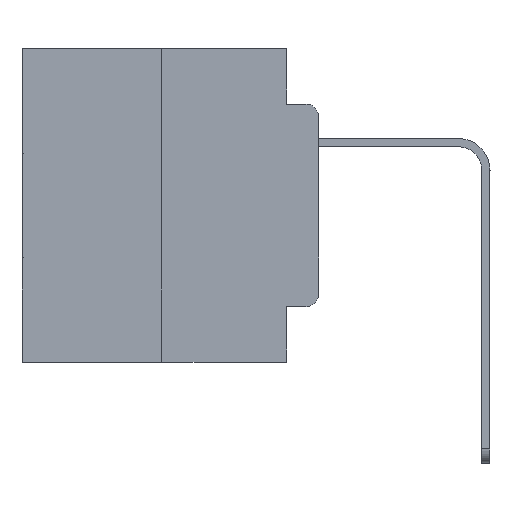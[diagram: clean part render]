
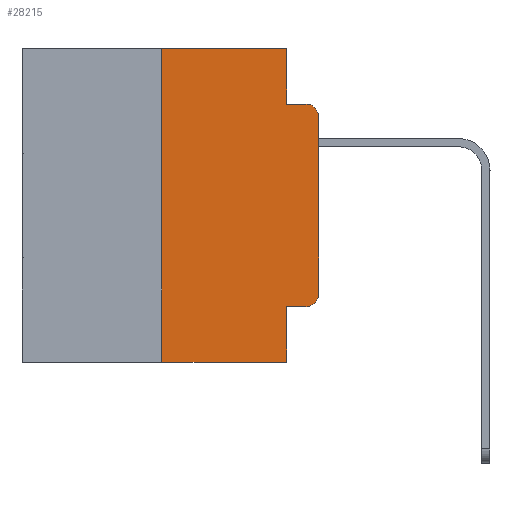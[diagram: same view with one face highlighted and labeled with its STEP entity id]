
A CAD part, left-side view. The second image highlights one B-rep face of the part: STEP entity #28215.
In plain terms, the highlighted planar face has unit normal (-1, 0, 0).
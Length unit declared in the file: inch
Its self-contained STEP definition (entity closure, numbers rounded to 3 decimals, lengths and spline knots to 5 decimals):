
#112 = EDGE_CURVE ( 'NONE', #27044, #25898, #26997, .T. ) ;
#832 = LINE ( 'NONE', #19827, #20653 ) ;
#1690 = EDGE_CURVE ( 'NONE', #2516, #24879, #832, .T. ) ;
#1736 = DIRECTION ( 'NONE',  ( 0., -1., 0. ) ) ;
#2111 = DIRECTION ( 'NONE',  ( -1., 0., 0. ) ) ;
#2393 = ORIENTED_EDGE ( 'NONE', *, *, #22960, .F. ) ;
#2516 = VERTEX_POINT ( 'NONE', #17266 ) ;
#3282 = ORIENTED_EDGE ( 'NONE', *, *, #7431, .T. ) ;
#4495 = EDGE_CURVE ( 'NONE', #27174, #2516, #18961, .T. ) ;
#4575 = VECTOR ( 'NONE', #15399, 39.37008 ) ;
#4580 = EDGE_LOOP ( 'NONE', ( #23330, #15863, #2393, #24850, #11859, #18437, #3282, #28692, #13666, #14845 ) ) ;
#4769 = CIRCLE ( 'NONE', #19741, 0.02 ) ;
#4883 = DIRECTION ( 'NONE',  ( 0., 0., -1. ) ) ;
#5229 = LINE ( 'NONE', #28736, #9497 ) ;
#5257 = DIRECTION ( 'NONE',  ( 0., 0., -1. ) ) ;
#5318 = EDGE_CURVE ( 'NONE', #24879, #15715, #4769, .T. ) ;
#5664 = CARTESIAN_POINT ( 'NONE',  ( 0., 0.25, 0. ) ) ;
#6042 = FACE_OUTER_BOUND ( 'NONE', #4580, .T. ) ;
#6263 = CARTESIAN_POINT ( 'NONE',  ( 0., 0.02, -0.3915 ) ) ;
#7431 = EDGE_CURVE ( 'NONE', #27044, #11054, #16066, .T. ) ;
#8309 = DIRECTION ( 'NONE',  ( 0., -1., 0. ) ) ;
#8562 = VECTOR ( 'NONE', #16497, 39.37008 ) ;
#8965 = VERTEX_POINT ( 'NONE', #24723 ) ;
#9441 = CARTESIAN_POINT ( 'NONE',  ( 0., 0.02, -0.1085 ) ) ;
#9497 = VECTOR ( 'NONE', #1736, 39.37008 ) ;
#9524 = DIRECTION ( 'NONE',  ( 1., 0., 0. ) ) ;
#9821 = DIRECTION ( 'NONE',  ( 0., -1., 0. ) ) ;
#10294 = DIRECTION ( 'NONE',  ( 0., 0., 1. ) ) ;
#11054 = VERTEX_POINT ( 'NONE', #13737 ) ;
#11495 = VECTOR ( 'NONE', #10294, 39.37008 ) ;
#11859 = ORIENTED_EDGE ( 'NONE', *, *, #14118, .F. ) ;
#12134 = LINE ( 'NONE', #14718, #8562 ) ;
#12325 = VERTEX_POINT ( 'NONE', #26578 ) ;
#12996 = CARTESIAN_POINT ( 'NONE',  ( 0., 0.02, -0.0885 ) ) ;
#13230 = EDGE_CURVE ( 'NONE', #14450, #11054, #27141, .T. ) ;
#13561 = CARTESIAN_POINT ( 'NONE',  ( 0., 0., -0.1085 ) ) ;
#13585 = VECTOR ( 'NONE', #17124, 39.37008 ) ;
#13666 = ORIENTED_EDGE ( 'NONE', *, *, #21667, .T. ) ;
#13737 = CARTESIAN_POINT ( 'NONE',  ( 0., 0.051, -0.5 ) ) ;
#14118 = EDGE_CURVE ( 'NONE', #25898, #8965, #28772, .T. ) ;
#14450 = VERTEX_POINT ( 'NONE', #20562 ) ;
#14718 = CARTESIAN_POINT ( 'NONE',  ( 0., 0.051, 0. ) ) ;
#14845 = ORIENTED_EDGE ( 'NONE', *, *, #4495, .T. ) ;
#14848 = CARTESIAN_POINT ( 'NONE',  ( 0., 0.25, -0.5 ) ) ;
#15038 = CARTESIAN_POINT ( 'NONE',  ( 0., 0.051, -0.4115 ) ) ;
#15212 = LINE ( 'NONE', #15038, #16638 ) ;
#15399 = DIRECTION ( 'NONE',  ( 0., 0., -1. ) ) ;
#15715 = VERTEX_POINT ( 'NONE', #12996 ) ;
#15863 = ORIENTED_EDGE ( 'NONE', *, *, #5318, .T. ) ;
#16066 = LINE ( 'NONE', #25900, #13585 ) ;
#16497 = DIRECTION ( 'NONE',  ( 0., 0., -1. ) ) ;
#16638 = VECTOR ( 'NONE', #8309, 39.37008 ) ;
#16796 = CARTESIAN_POINT ( 'NONE',  ( 0., 0.25, 0. ) ) ;
#17124 = DIRECTION ( 'NONE',  ( 0., -1., 0. ) ) ;
#17266 = CARTESIAN_POINT ( 'NONE',  ( 0., 0., -0.3915 ) ) ;
#17420 = CARTESIAN_POINT ( 'NONE',  ( 0., 0.02, -0.4115 ) ) ;
#17970 = CARTESIAN_POINT ( 'NONE',  ( 0., 0.051, 0. ) ) ;
#18437 = ORIENTED_EDGE ( 'NONE', *, *, #112, .F. ) ;
#18443 = DIRECTION ( 'NONE',  ( -1., 0., 0. ) ) ;
#18961 = CIRCLE ( 'NONE', #26318, 0.02 ) ;
#18964 = VECTOR ( 'NONE', #9821, 39.37008 ) ;
#19741 = AXIS2_PLACEMENT_3D ( 'NONE', #9441, #18443, #4883 ) ;
#19827 = CARTESIAN_POINT ( 'NONE',  ( 0., 0., 0. ) ) ;
#20153 = EDGE_CURVE ( 'NONE', #8965, #12325, #12134, .T. ) ;
#20562 = CARTESIAN_POINT ( 'NONE',  ( 0., 0.051, -0.4115 ) ) ;
#20653 = VECTOR ( 'NONE', #24332, 39.37008 ) ;
#21667 = EDGE_CURVE ( 'NONE', #14450, #27174, #15212, .T. ) ;
#22438 = DIRECTION ( 'NONE',  ( 0., 0., -1. ) ) ;
#22960 = EDGE_CURVE ( 'NONE', #12325, #15715, #5229, .T. ) ;
#23330 = ORIENTED_EDGE ( 'NONE', *, *, #1690, .T. ) ;
#23427 = CARTESIAN_POINT ( 'NONE',  ( 0., 0.473, 0. ) ) ;
#24332 = DIRECTION ( 'NONE',  ( 0., 0., 1. ) ) ;
#24723 = CARTESIAN_POINT ( 'NONE',  ( 0., 0.051, 0. ) ) ;
#24850 = ORIENTED_EDGE ( 'NONE', *, *, #20153, .F. ) ;
#24879 = VERTEX_POINT ( 'NONE', #13561 ) ;
#25761 = AXIS2_PLACEMENT_3D ( 'NONE', #23427, #9524, #5257 ) ;
#25784 = CARTESIAN_POINT ( 'NONE',  ( 0., 0.473, 0. ) ) ;
#25898 = VERTEX_POINT ( 'NONE', #16796 ) ;
#25900 = CARTESIAN_POINT ( 'NONE',  ( 0., 0.473, -0.5 ) ) ;
#26318 = AXIS2_PLACEMENT_3D ( 'NONE', #6263, #2111, #22438 ) ;
#26578 = CARTESIAN_POINT ( 'NONE',  ( 0., 0.051, -0.0885 ) ) ;
#26997 = LINE ( 'NONE', #5664, #11495 ) ;
#27044 = VERTEX_POINT ( 'NONE', #14848 ) ;
#27141 = LINE ( 'NONE', #17970, #4575 ) ;
#27174 = VERTEX_POINT ( 'NONE', #17420 ) ;
#27630 = PLANE ( 'NONE',  #25761 ) ;
#28215 = ADVANCED_FACE ( 'NONE', ( #6042 ), #27630, .F. ) ;
#28692 = ORIENTED_EDGE ( 'NONE', *, *, #13230, .F. ) ;
#28736 = CARTESIAN_POINT ( 'NONE',  ( 0., 0.051, -0.0885 ) ) ;
#28772 = LINE ( 'NONE', #25784, #18964 ) ;
